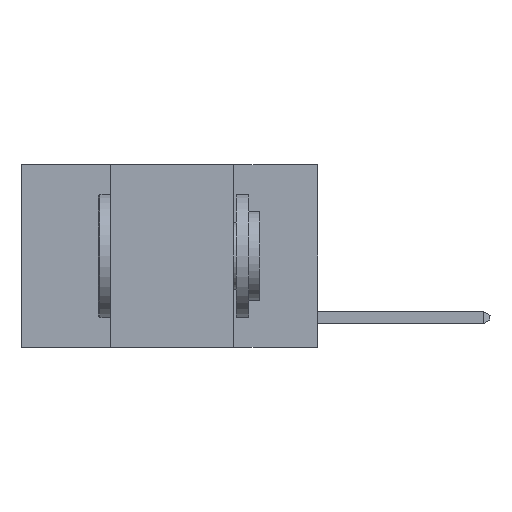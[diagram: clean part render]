
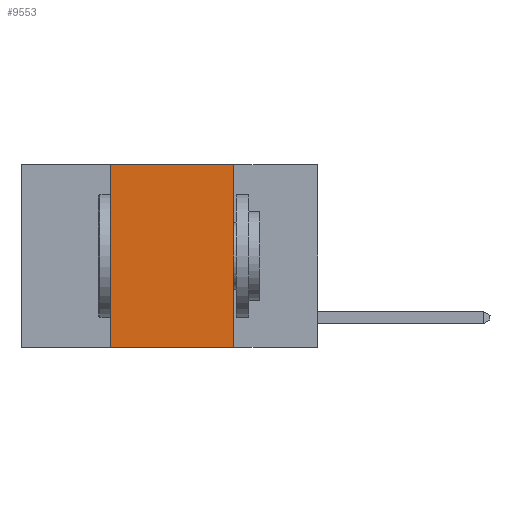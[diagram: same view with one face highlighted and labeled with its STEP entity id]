
A CAD part, left-side view. The second image highlights one B-rep face of the part: STEP entity #9553.
In plain terms, the highlighted planar face has unit normal (-1, 0, 0).
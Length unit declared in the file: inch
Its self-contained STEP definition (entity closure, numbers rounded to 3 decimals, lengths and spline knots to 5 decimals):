
#790 = FACE_OUTER_BOUND ( 'NONE', #1393, .T. ) ;
#1004 = LINE ( 'NONE', #5650, #11657 ) ;
#1393 = EDGE_LOOP ( 'NONE', ( #8773, #3172, #2316, #5805 ) ) ;
#1469 = CARTESIAN_POINT ( 'NONE',  ( 0., 0.42, -0.37 ) ) ;
#1938 = DIRECTION ( 'NONE',  ( 1., 0., 0. ) ) ;
#2316 = ORIENTED_EDGE ( 'NONE', *, *, #12342, .F. ) ;
#3172 = ORIENTED_EDGE ( 'NONE', *, *, #12469, .F. ) ;
#3318 = LINE ( 'NONE', #9368, #13747 ) ;
#3844 = LINE ( 'NONE', #4916, #9559 ) ;
#4916 = CARTESIAN_POINT ( 'NONE',  ( 0., 0.17, 0. ) ) ;
#4964 = EDGE_CURVE ( 'NONE', #6512, #9884, #1004, .T. ) ;
#5046 = CARTESIAN_POINT ( 'NONE',  ( 0., 0.17, -0.37 ) ) ;
#5650 = CARTESIAN_POINT ( 'NONE',  ( 0., 0.6, -0.37 ) ) ;
#5661 = VECTOR ( 'NONE', #6816, 39.37008 ) ;
#5805 = ORIENTED_EDGE ( 'NONE', *, *, #4964, .T. ) ;
#6512 = VERTEX_POINT ( 'NONE', #1469 ) ;
#6816 = DIRECTION ( 'NONE',  ( 0., 0., 1. ) ) ;
#7344 = VERTEX_POINT ( 'NONE', #7470 ) ;
#7470 = CARTESIAN_POINT ( 'NONE',  ( 0., 0.17, 0. ) ) ;
#8773 = ORIENTED_EDGE ( 'NONE', *, *, #11208, .F. ) ;
#8903 = PLANE ( 'NONE',  #9504 ) ;
#9368 = CARTESIAN_POINT ( 'NONE',  ( 0., 0.6, 0. ) ) ;
#9504 = AXIS2_PLACEMENT_3D ( 'NONE', #10045, #1938, #12428 ) ;
#9553 = ADVANCED_FACE ( 'NONE', ( #790 ), #8903, .F. ) ;
#9559 = VECTOR ( 'NONE', #10739, 39.37008 ) ;
#9884 = VERTEX_POINT ( 'NONE', #5046 ) ;
#10045 = CARTESIAN_POINT ( 'NONE',  ( 0., 0.6, 0. ) ) ;
#10739 = DIRECTION ( 'NONE',  ( 0., 0., -1. ) ) ;
#11208 = EDGE_CURVE ( 'NONE', #7344, #9884, #3844, .T. ) ;
#11657 = VECTOR ( 'NONE', #14506, 39.37008 ) ;
#12342 = EDGE_CURVE ( 'NONE', #6512, #12458, #14974, .T. ) ;
#12428 = DIRECTION ( 'NONE',  ( 0., 0., -1. ) ) ;
#12458 = VERTEX_POINT ( 'NONE', #15116 ) ;
#12469 = EDGE_CURVE ( 'NONE', #12458, #7344, #3318, .T. ) ;
#13747 = VECTOR ( 'NONE', #13812, 39.37008 ) ;
#13812 = DIRECTION ( 'NONE',  ( 0., -1., 0. ) ) ;
#14506 = DIRECTION ( 'NONE',  ( 0., -1., 0. ) ) ;
#14974 = LINE ( 'NONE', #15045, #5661 ) ;
#15045 = CARTESIAN_POINT ( 'NONE',  ( 0., 0.42, 0. ) ) ;
#15116 = CARTESIAN_POINT ( 'NONE',  ( 0., 0.42, 0. ) ) ;
